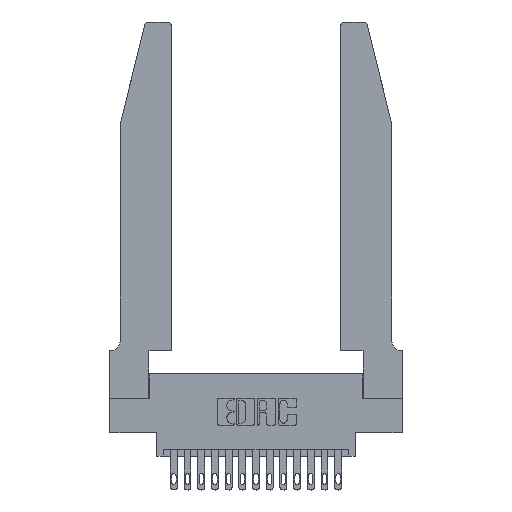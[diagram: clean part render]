
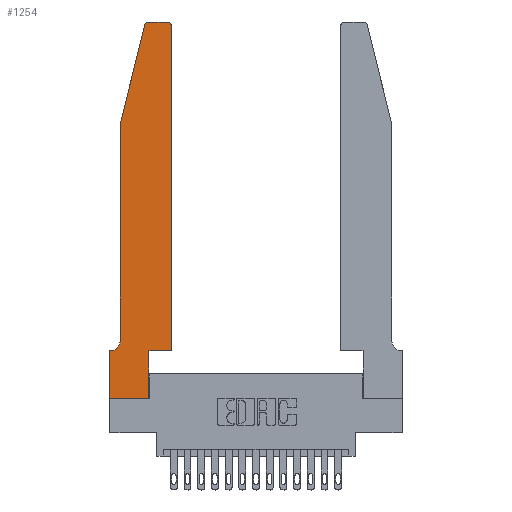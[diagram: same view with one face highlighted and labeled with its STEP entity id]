
A CAD part, top view. The second image highlights one B-rep face of the part: STEP entity #1254.
In plain terms, the highlighted planar face has unit normal (0, 0, 1).
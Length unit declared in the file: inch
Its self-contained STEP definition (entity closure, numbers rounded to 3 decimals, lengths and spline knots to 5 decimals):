
#23 = VECTOR ( 'NONE', #9965, 39.37008 ) ;
#429 = DIRECTION ( 'NONE',  ( 1., 0., 0. ) ) ;
#897 = VECTOR ( 'NONE', #15516, 39.37008 ) ;
#997 = DIRECTION ( 'NONE',  ( 1., 0., 0. ) ) ;
#1036 = VECTOR ( 'NONE', #7252, 39.37008 ) ;
#1065 = ORIENTED_EDGE ( 'NONE', *, *, #16843, .T. ) ;
#1254 = ADVANCED_FACE ( 'NONE', ( #13733 ), #17118, .T. ) ;
#1334 = ORIENTED_EDGE ( 'NONE', *, *, #2424, .T. ) ;
#1401 = CIRCLE ( 'NONE', #14164, 0.07 ) ;
#1648 = ORIENTED_EDGE ( 'NONE', *, *, #15320, .T. ) ;
#1677 = ORIENTED_EDGE ( 'NONE', *, *, #13444, .T. ) ;
#1743 = CARTESIAN_POINT ( 'NONE',  ( 0.0055, 0.42, 0.37 ) ) ;
#1757 = CARTESIAN_POINT ( 'NONE',  ( 0.284, 2.72, 0.37 ) ) ;
#1801 = LINE ( 'NONE', #6110, #14848 ) ;
#1820 = DIRECTION ( 'NONE',  ( 1., 0., 0. ) ) ;
#2016 = AXIS2_PLACEMENT_3D ( 'NONE', #9753, #2518, #997 ) ;
#2413 = ORIENTED_EDGE ( 'NONE', *, *, #6428, .T. ) ;
#2424 = EDGE_CURVE ( 'NONE', #11962, #6484, #5459, .T. ) ;
#2434 = ORIENTED_EDGE ( 'NONE', *, *, #16907, .T. ) ;
#2518 = DIRECTION ( 'NONE',  ( 0., 0., 1. ) ) ;
#2715 = EDGE_CURVE ( 'NONE', #14951, #16789, #12543, .T. ) ;
#2753 = CARTESIAN_POINT ( 'NONE',  ( 0.4205, 2.75, 0.37 ) ) ;
#2823 = VECTOR ( 'NONE', #8852, 39.37008 ) ;
#2918 = VERTEX_POINT ( 'NONE', #14240 ) ;
#3013 = VERTEX_POINT ( 'NONE', #13003 ) ;
#3215 = CARTESIAN_POINT ( 'NONE',  ( 0.0755, 2., 0.37 ) ) ;
#3855 = EDGE_CURVE ( 'NONE', #12509, #9257, #5646, .T. ) ;
#4456 = CARTESIAN_POINT ( 'NONE',  ( 0., 0., 0.37 ) ) ;
#4771 = DIRECTION ( 'NONE',  ( 0., -1., 0. ) ) ;
#4819 = DIRECTION ( 'NONE',  ( -1., 0., 0. ) ) ;
#4947 = ORIENTED_EDGE ( 'NONE', *, *, #3855, .T. ) ;
#5298 = EDGE_CURVE ( 'NONE', #16789, #6541, #17731, .T. ) ;
#5459 = LINE ( 'NONE', #7746, #7512 ) ;
#5646 = LINE ( 'NONE', #17943, #15491 ) ;
#5838 = CARTESIAN_POINT ( 'NONE',  ( 0.4505, 0.35, 0.37 ) ) ;
#5862 = AXIS2_PLACEMENT_3D ( 'NONE', #17337, #13542, #14943 ) ;
#6110 = CARTESIAN_POINT ( 'NONE',  ( 0., 0., 0.37 ) ) ;
#6174 = VERTEX_POINT ( 'NONE', #6499 ) ;
#6428 = EDGE_CURVE ( 'NONE', #9257, #14951, #1801, .T. ) ;
#6484 = VERTEX_POINT ( 'NONE', #11865 ) ;
#6499 = CARTESIAN_POINT ( 'NONE',  ( 0.25487, 2.72718, 0.37 ) ) ;
#6541 = VERTEX_POINT ( 'NONE', #6862 ) ;
#6862 = CARTESIAN_POINT ( 'NONE',  ( 0.4505, 0.35, 0.37 ) ) ;
#7010 = ORIENTED_EDGE ( 'NONE', *, *, #7168, .T. ) ;
#7168 = EDGE_CURVE ( 'NONE', #17880, #18683, #15279, .T. ) ;
#7252 = DIRECTION ( 'NONE',  ( 1., 0., 0. ) ) ;
#7417 = LINE ( 'NONE', #7509, #16805 ) ;
#7509 = CARTESIAN_POINT ( 'NONE',  ( 0.0755, 2., 0.37 ) ) ;
#7512 = VECTOR ( 'NONE', #17499, 39.37008 ) ;
#7633 = DIRECTION ( 'NONE',  ( 0., 0., 1. ) ) ;
#7746 = CARTESIAN_POINT ( 'NONE',  ( 0.0755, 2., 0.37 ) ) ;
#7779 = LINE ( 'NONE', #14262, #23 ) ;
#8163 = CARTESIAN_POINT ( 'NONE',  ( 0.2865, 0.35, 0.37 ) ) ;
#8852 = DIRECTION ( 'NONE',  ( -1., 0., 0. ) ) ;
#9015 = LINE ( 'NONE', #14924, #2823 ) ;
#9030 = DIRECTION ( 'NONE',  ( 0., 0., -1. ) ) ;
#9124 = AXIS2_PLACEMENT_3D ( 'NONE', #1757, #7633, #1820 ) ;
#9257 = VERTEX_POINT ( 'NONE', #4456 ) ;
#9753 = CARTESIAN_POINT ( 'NONE',  ( 0., 0.35, 0.37 ) ) ;
#9965 = DIRECTION ( 'NONE',  ( 0., 1., 0. ) ) ;
#10760 = DIRECTION ( 'NONE',  ( -0.239, -0.971, 0. ) ) ;
#11103 = ORIENTED_EDGE ( 'NONE', *, *, #5298, .T. ) ;
#11466 = EDGE_CURVE ( 'NONE', #6484, #2918, #1401, .T. ) ;
#11665 = ORIENTED_EDGE ( 'NONE', *, *, #12224, .T. ) ;
#11810 = CARTESIAN_POINT ( 'NONE',  ( 0.4505, 2.72, 0.37 ) ) ;
#11865 = CARTESIAN_POINT ( 'NONE',  ( 0.0755, 0.42, 0.37 ) ) ;
#11962 = VERTEX_POINT ( 'NONE', #3215 ) ;
#12224 = EDGE_CURVE ( 'NONE', #6541, #17880, #7779, .T. ) ;
#12262 = EDGE_LOOP ( 'NONE', ( #1065, #1648, #2434, #1334, #13348, #1677, #4947, #2413, #15865, #11103, #11665, #7010 ) ) ;
#12509 = VERTEX_POINT ( 'NONE', #14773 ) ;
#12543 = LINE ( 'NONE', #8163, #897 ) ;
#12771 = VECTOR ( 'NONE', #4819, 39.37008 ) ;
#13003 = CARTESIAN_POINT ( 'NONE',  ( 0.284, 2.75, 0.37 ) ) ;
#13348 = ORIENTED_EDGE ( 'NONE', *, *, #11466, .T. ) ;
#13444 = EDGE_CURVE ( 'NONE', #2918, #12509, #17142, .T. ) ;
#13542 = DIRECTION ( 'NONE',  ( 0., 0., 1. ) ) ;
#13733 = FACE_OUTER_BOUND ( 'NONE', #12262, .T. ) ;
#14164 = AXIS2_PLACEMENT_3D ( 'NONE', #1743, #9030, #16387 ) ;
#14240 = CARTESIAN_POINT ( 'NONE',  ( 0.0055, 0.35, 0.37 ) ) ;
#14262 = CARTESIAN_POINT ( 'NONE',  ( 0.4505, 0.35, 0.37 ) ) ;
#14773 = CARTESIAN_POINT ( 'NONE',  ( 0., 0.35, 0.37 ) ) ;
#14848 = VECTOR ( 'NONE', #429, 39.37008 ) ;
#14924 = CARTESIAN_POINT ( 'NONE',  ( 0.2605, 2.75, 0.37 ) ) ;
#14943 = DIRECTION ( 'NONE',  ( 1., 0., 0. ) ) ;
#14951 = VERTEX_POINT ( 'NONE', #17200 ) ;
#15279 = CIRCLE ( 'NONE', #5862, 0.03 ) ;
#15320 = EDGE_CURVE ( 'NONE', #3013, #6174, #17967, .T. ) ;
#15491 = VECTOR ( 'NONE', #4771, 39.37008 ) ;
#15516 = DIRECTION ( 'NONE',  ( 0., 1., 0. ) ) ;
#15865 = ORIENTED_EDGE ( 'NONE', *, *, #2715, .T. ) ;
#16091 = CARTESIAN_POINT ( 'NONE',  ( 0.2865, 0.35, 0.37 ) ) ;
#16387 = DIRECTION ( 'NONE',  ( -1., 0., 0. ) ) ;
#16789 = VERTEX_POINT ( 'NONE', #16091 ) ;
#16805 = VECTOR ( 'NONE', #10760, 39.37008 ) ;
#16843 = EDGE_CURVE ( 'NONE', #18683, #3013, #9015, .T. ) ;
#16907 = EDGE_CURVE ( 'NONE', #6174, #11962, #7417, .T. ) ;
#17118 = PLANE ( 'NONE',  #2016 ) ;
#17142 = LINE ( 'NONE', #17933, #12771 ) ;
#17200 = CARTESIAN_POINT ( 'NONE',  ( 0.2865, 0., 0.37 ) ) ;
#17337 = CARTESIAN_POINT ( 'NONE',  ( 0.4205, 2.72, 0.37 ) ) ;
#17499 = DIRECTION ( 'NONE',  ( 0., -1., 0. ) ) ;
#17731 = LINE ( 'NONE', #5838, #1036 ) ;
#17880 = VERTEX_POINT ( 'NONE', #11810 ) ;
#17933 = CARTESIAN_POINT ( 'NONE',  ( 0.0755, 0.35, 0.37 ) ) ;
#17943 = CARTESIAN_POINT ( 'NONE',  ( 0., 0., 0.37 ) ) ;
#17967 = CIRCLE ( 'NONE', #9124, 0.03 ) ;
#18683 = VERTEX_POINT ( 'NONE', #2753 ) ;
